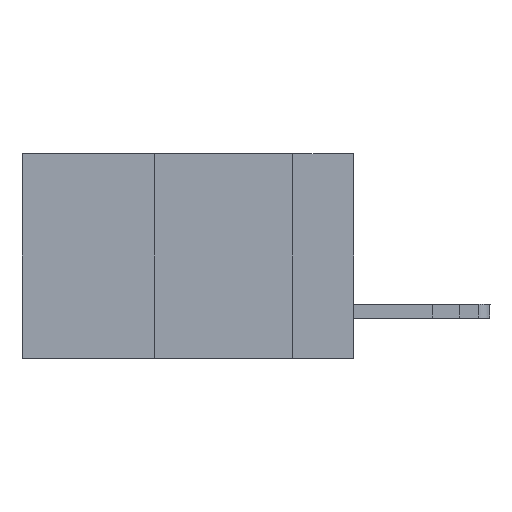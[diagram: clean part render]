
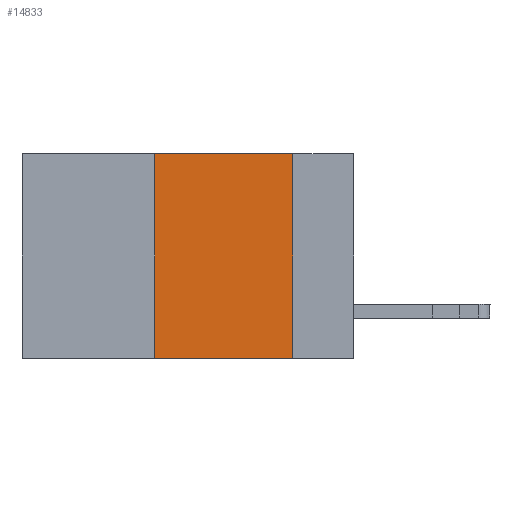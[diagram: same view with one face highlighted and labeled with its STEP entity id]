
A CAD part, left-side view. The second image highlights one B-rep face of the part: STEP entity #14833.
In plain terms, the highlighted planar face has unit normal (-1, 0, 0).
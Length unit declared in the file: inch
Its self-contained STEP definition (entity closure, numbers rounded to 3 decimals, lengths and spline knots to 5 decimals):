
#1393 = ORIENTED_EDGE ( 'NONE', *, *, #25374, .T. ) ;
#1519 = ORIENTED_EDGE ( 'NONE', *, *, #26333, .F. ) ;
#4678 = CARTESIAN_POINT ( 'NONE',  ( 0., 0.11, -0.37 ) ) ;
#4896 = DIRECTION ( 'NONE',  ( 0., 0., 1. ) ) ;
#5972 = DIRECTION ( 'NONE',  ( 0., 0., -1. ) ) ;
#6061 = ORIENTED_EDGE ( 'NONE', *, *, #20742, .F. ) ;
#6671 = CARTESIAN_POINT ( 'NONE',  ( 0., 0.11, 0. ) ) ;
#7488 = LINE ( 'NONE', #21362, #24256 ) ;
#8243 = CARTESIAN_POINT ( 'NONE',  ( 0., 0.11, 0. ) ) ;
#9432 = PLANE ( 'NONE',  #26939 ) ;
#11366 = DIRECTION ( 'NONE',  ( 0., -1., 0. ) ) ;
#11415 = DIRECTION ( 'NONE',  ( 1., 0., 0. ) ) ;
#13667 = CARTESIAN_POINT ( 'NONE',  ( 0., 0.6, 0. ) ) ;
#13881 = CARTESIAN_POINT ( 'NONE',  ( 0., 0.36, 0. ) ) ;
#14833 = ADVANCED_FACE ( 'NONE', ( #27945 ), #9432, .F. ) ;
#15339 = VERTEX_POINT ( 'NONE', #19106 ) ;
#15596 = CARTESIAN_POINT ( 'NONE',  ( 0., 0.6, -0.37 ) ) ;
#16678 = DIRECTION ( 'NONE',  ( 0., -1., 0. ) ) ;
#17007 = VERTEX_POINT ( 'NONE', #6671 ) ;
#17554 = ORIENTED_EDGE ( 'NONE', *, *, #17929, .F. ) ;
#17929 = EDGE_CURVE ( 'NONE', #17007, #24665, #24513, .T. ) ;
#18012 = VECTOR ( 'NONE', #11366, 39.37008 ) ;
#18597 = CARTESIAN_POINT ( 'NONE',  ( 0., 0.36, 0. ) ) ;
#19106 = CARTESIAN_POINT ( 'NONE',  ( 0., 0.36, -0.37 ) ) ;
#19138 = VECTOR ( 'NONE', #5972, 39.37008 ) ;
#20105 = VECTOR ( 'NONE', #4896, 39.37008 ) ;
#20600 = DIRECTION ( 'NONE',  ( 0., 0., -1. ) ) ;
#20742 = EDGE_CURVE ( 'NONE', #23698, #17007, #7488, .T. ) ;
#21362 = CARTESIAN_POINT ( 'NONE',  ( 0., 0.6, 0. ) ) ;
#23698 = VERTEX_POINT ( 'NONE', #13881 ) ;
#24256 = VECTOR ( 'NONE', #16678, 39.37008 ) ;
#24513 = LINE ( 'NONE', #8243, #19138 ) ;
#24665 = VERTEX_POINT ( 'NONE', #4678 ) ;
#25374 = EDGE_CURVE ( 'NONE', #15339, #24665, #29463, .T. ) ;
#26333 = EDGE_CURVE ( 'NONE', #15339, #23698, #28091, .T. ) ;
#26939 = AXIS2_PLACEMENT_3D ( 'NONE', #13667, #11415, #20600 ) ;
#27945 = FACE_OUTER_BOUND ( 'NONE', #29399, .T. ) ;
#28091 = LINE ( 'NONE', #18597, #20105 ) ;
#29399 = EDGE_LOOP ( 'NONE', ( #17554, #6061, #1519, #1393 ) ) ;
#29463 = LINE ( 'NONE', #15596, #18012 ) ;
